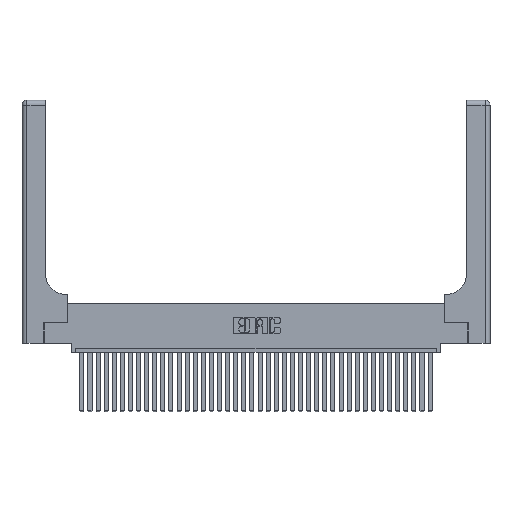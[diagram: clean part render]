
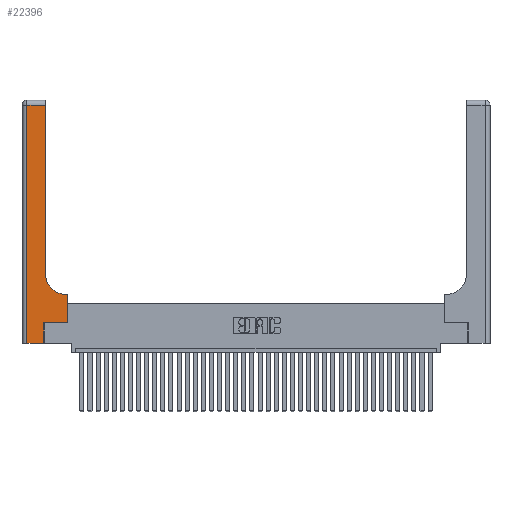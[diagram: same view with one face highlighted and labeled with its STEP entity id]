
A CAD part, top view. The second image highlights one B-rep face of the part: STEP entity #22396.
In plain terms, the highlighted planar face has unit normal (0, 0, 1).
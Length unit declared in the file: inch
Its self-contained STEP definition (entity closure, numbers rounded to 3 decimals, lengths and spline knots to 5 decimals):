
#443 = CARTESIAN_POINT ( 'NONE',  ( 0.2915, 2.94, 0.37 ) ) ;
#2438 = LINE ( 'NONE', #25008, #30002 ) ;
#2646 = VECTOR ( 'NONE', #23639, 39.37008 ) ;
#2967 = VECTOR ( 'NONE', #3718, 39.37008 ) ;
#2977 = DIRECTION ( 'NONE',  ( 0., 1., 0. ) ) ;
#3718 = DIRECTION ( 'NONE',  ( -1., 0., 0. ) ) ;
#3740 = ORIENTED_EDGE ( 'NONE', *, *, #31376, .T. ) ;
#3878 = LINE ( 'NONE', #33223, #33270 ) ;
#3913 = LINE ( 'NONE', #14321, #37870 ) ;
#4123 = LINE ( 'NONE', #30838, #5791 ) ;
#5791 = VECTOR ( 'NONE', #13238, 39.37008 ) ;
#7830 = FACE_OUTER_BOUND ( 'NONE', #26738, .T. ) ;
#8166 = EDGE_CURVE ( 'NONE', #30021, #13437, #13260, .T. ) ;
#8322 = CARTESIAN_POINT ( 'NONE',  ( 0.269, 0., 0.37 ) ) ;
#10523 = CARTESIAN_POINT ( 'NONE',  ( 0., 3., 0.37 ) ) ;
#10741 = AXIS2_PLACEMENT_3D ( 'NONE', #10523, #31109, #25291 ) ;
#10961 = EDGE_CURVE ( 'NONE', #13437, #26378, #3878, .T. ) ;
#11739 = LINE ( 'NONE', #22345, #37437 ) ;
#12618 = CARTESIAN_POINT ( 'NONE',  ( 0.5585, 0.6, 0.37 ) ) ;
#13238 = DIRECTION ( 'NONE',  ( 0., 1., 0. ) ) ;
#13260 = LINE ( 'NONE', #34646, #2646 ) ;
#13302 = VERTEX_POINT ( 'NONE', #34941 ) ;
#13325 = DIRECTION ( 'NONE',  ( -1., 0., 0. ) ) ;
#13437 = VERTEX_POINT ( 'NONE', #36213 ) ;
#13722 = VERTEX_POINT ( 'NONE', #35213 ) ;
#14144 = CARTESIAN_POINT ( 'NONE',  ( 0.269, 0., 0.37 ) ) ;
#14263 = DIRECTION ( 'NONE',  ( 0., 1., 0. ) ) ;
#14321 = CARTESIAN_POINT ( 'NONE',  ( 0.5585, 0.25, 0.37 ) ) ;
#14755 = VERTEX_POINT ( 'NONE', #443 ) ;
#16363 = LINE ( 'NONE', #32727, #2967 ) ;
#16510 = ORIENTED_EDGE ( 'NONE', *, *, #17588, .T. ) ;
#17588 = EDGE_CURVE ( 'NONE', #13302, #14755, #4123, .T. ) ;
#18597 = DIRECTION ( 'NONE',  ( 1., 0., 0. ) ) ;
#20682 = ORIENTED_EDGE ( 'NONE', *, *, #33602, .T. ) ;
#22327 = LINE ( 'NONE', #14144, #33764 ) ;
#22345 = CARTESIAN_POINT ( 'NONE',  ( 0.269, 0.25, 0.37 ) ) ;
#22396 = ADVANCED_FACE ( 'NONE', ( #7830 ), #28134, .F. ) ;
#23142 = CARTESIAN_POINT ( 'NONE',  ( 0.06, 2.94, 0.37 ) ) ;
#23525 = ORIENTED_EDGE ( 'NONE', *, *, #26792, .T. ) ;
#23639 = DIRECTION ( 'NONE',  ( 0., -1., 0. ) ) ;
#23719 = CARTESIAN_POINT ( 'NONE',  ( 0.5585, 0.25, 0.37 ) ) ;
#24631 = VERTEX_POINT ( 'NONE', #25198 ) ;
#25008 = CARTESIAN_POINT ( 'NONE',  ( 0.2915, 0.6, 0.37 ) ) ;
#25198 = CARTESIAN_POINT ( 'NONE',  ( 0.5415, 0.6, 0.37 ) ) ;
#25291 = DIRECTION ( 'NONE',  ( -1., 0., 0. ) ) ;
#26020 = ORIENTED_EDGE ( 'NONE', *, *, #35733, .T. ) ;
#26378 = VERTEX_POINT ( 'NONE', #8322 ) ;
#26738 = EDGE_LOOP ( 'NONE', ( #16510, #3740, #33171, #37304, #34270, #29762, #20682, #26020, #23525 ) ) ;
#26785 = VERTEX_POINT ( 'NONE', #12618 ) ;
#26792 = EDGE_CURVE ( 'NONE', #24631, #13302, #36358, .T. ) ;
#27335 = AXIS2_PLACEMENT_3D ( 'NONE', #29818, #27411, #29953 ) ;
#27411 = DIRECTION ( 'NONE',  ( 0., 0., -1. ) ) ;
#28134 = PLANE ( 'NONE',  #10741 ) ;
#28150 = VERTEX_POINT ( 'NONE', #23719 ) ;
#29762 = ORIENTED_EDGE ( 'NONE', *, *, #33457, .T. ) ;
#29818 = CARTESIAN_POINT ( 'NONE',  ( 0.5415, 0.85, 0.37 ) ) ;
#29953 = DIRECTION ( 'NONE',  ( 1., 0., 0. ) ) ;
#30002 = VECTOR ( 'NONE', #13325, 39.37008 ) ;
#30021 = VERTEX_POINT ( 'NONE', #23142 ) ;
#30838 = CARTESIAN_POINT ( 'NONE',  ( 0.2915, 3., 0.37 ) ) ;
#31109 = DIRECTION ( 'NONE',  ( 0., 0., -1. ) ) ;
#31376 = EDGE_CURVE ( 'NONE', #14755, #30021, #16363, .T. ) ;
#31874 = EDGE_CURVE ( 'NONE', #26378, #13722, #22327, .T. ) ;
#32727 = CARTESIAN_POINT ( 'NONE',  ( 0., 2.94, 0.37 ) ) ;
#33171 = ORIENTED_EDGE ( 'NONE', *, *, #8166, .T. ) ;
#33223 = CARTESIAN_POINT ( 'NONE',  ( 0., 0., 0.37 ) ) ;
#33270 = VECTOR ( 'NONE', #18597, 39.37008 ) ;
#33457 = EDGE_CURVE ( 'NONE', #13722, #28150, #11739, .T. ) ;
#33602 = EDGE_CURVE ( 'NONE', #28150, #26785, #3913, .T. ) ;
#33764 = VECTOR ( 'NONE', #14263, 39.37008 ) ;
#34080 = DIRECTION ( 'NONE',  ( 1., 0., 0. ) ) ;
#34270 = ORIENTED_EDGE ( 'NONE', *, *, #31874, .T. ) ;
#34646 = CARTESIAN_POINT ( 'NONE',  ( 0.06, 3., 0.37 ) ) ;
#34941 = CARTESIAN_POINT ( 'NONE',  ( 0.2915, 0.85, 0.37 ) ) ;
#35213 = CARTESIAN_POINT ( 'NONE',  ( 0.269, 0.25, 0.37 ) ) ;
#35733 = EDGE_CURVE ( 'NONE', #26785, #24631, #2438, .T. ) ;
#36213 = CARTESIAN_POINT ( 'NONE',  ( 0.06, 0., 0.37 ) ) ;
#36358 = CIRCLE ( 'NONE', #27335, 0.25 ) ;
#37304 = ORIENTED_EDGE ( 'NONE', *, *, #10961, .T. ) ;
#37437 = VECTOR ( 'NONE', #34080, 39.37008 ) ;
#37870 = VECTOR ( 'NONE', #2977, 39.37008 ) ;
